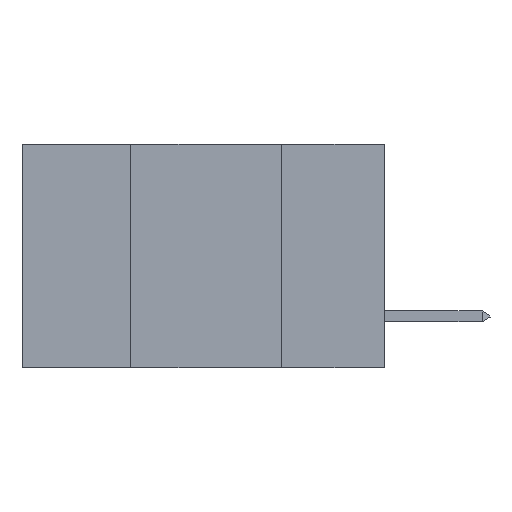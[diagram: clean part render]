
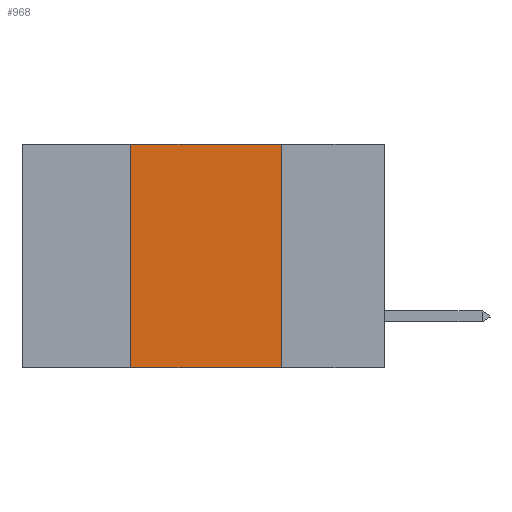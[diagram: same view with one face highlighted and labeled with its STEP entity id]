
A CAD part, left-side view. The second image highlights one B-rep face of the part: STEP entity #968.
In plain terms, the highlighted planar face has unit normal (-1, 0, 0).
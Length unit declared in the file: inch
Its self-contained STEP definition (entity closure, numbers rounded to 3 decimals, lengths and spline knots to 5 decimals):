
#968 = ADVANCED_FACE ( 'NONE', ( #14739 ), #27433, .F. ) ;
#1146 = EDGE_CURVE ( 'NONE', #17341, #30372, #25271, .T. ) ;
#1219 = CARTESIAN_POINT ( 'NONE',  ( 0., 0.42, -0.37 ) ) ;
#2249 = DIRECTION ( 'NONE',  ( 1., 0., 0. ) ) ;
#3747 = CARTESIAN_POINT ( 'NONE',  ( 0., 0.17, 0. ) ) ;
#4158 = DIRECTION ( 'NONE',  ( 0., -1., 0. ) ) ;
#4792 = DIRECTION ( 'NONE',  ( 0., 0., -1. ) ) ;
#5296 = LINE ( 'NONE', #9425, #22222 ) ;
#6341 = VERTEX_POINT ( 'NONE', #28883 ) ;
#7654 = ORIENTED_EDGE ( 'NONE', *, *, #20217, .T. ) ;
#8014 = CARTESIAN_POINT ( 'NONE',  ( 0., 0.42, 0. ) ) ;
#8727 = DIRECTION ( 'NONE',  ( 0., 0., 1. ) ) ;
#8892 = VECTOR ( 'NONE', #24467, 39.37008 ) ;
#9425 = CARTESIAN_POINT ( 'NONE',  ( 0., 0.6, -0.37 ) ) ;
#9540 = VERTEX_POINT ( 'NONE', #1219 ) ;
#10254 = CARTESIAN_POINT ( 'NONE',  ( 0., 0.6, 0. ) ) ;
#10966 = ORIENTED_EDGE ( 'NONE', *, *, #18745, .F. ) ;
#12131 = DIRECTION ( 'NONE',  ( 0., -1., 0. ) ) ;
#13094 = ORIENTED_EDGE ( 'NONE', *, *, #1146, .F. ) ;
#13785 = LINE ( 'NONE', #8014, #29041 ) ;
#14739 = FACE_OUTER_BOUND ( 'NONE', #22120, .T. ) ;
#14988 = LINE ( 'NONE', #26780, #16953 ) ;
#16953 = VECTOR ( 'NONE', #12131, 39.37008 ) ;
#17019 = CARTESIAN_POINT ( 'NONE',  ( 0., 0.17, -0.37 ) ) ;
#17341 = VERTEX_POINT ( 'NONE', #3747 ) ;
#18745 = EDGE_CURVE ( 'NONE', #6341, #17341, #14988, .T. ) ;
#19421 = AXIS2_PLACEMENT_3D ( 'NONE', #10254, #2249, #4792 ) ;
#19465 = EDGE_CURVE ( 'NONE', #9540, #6341, #13785, .T. ) ;
#20217 = EDGE_CURVE ( 'NONE', #9540, #30372, #5296, .T. ) ;
#22120 = EDGE_LOOP ( 'NONE', ( #13094, #10966, #24376, #7654 ) ) ;
#22222 = VECTOR ( 'NONE', #4158, 39.37008 ) ;
#24376 = ORIENTED_EDGE ( 'NONE', *, *, #19465, .F. ) ;
#24467 = DIRECTION ( 'NONE',  ( 0., 0., -1. ) ) ;
#25271 = LINE ( 'NONE', #26086, #8892 ) ;
#26086 = CARTESIAN_POINT ( 'NONE',  ( 0., 0.17, 0. ) ) ;
#26780 = CARTESIAN_POINT ( 'NONE',  ( 0., 0.6, 0. ) ) ;
#27433 = PLANE ( 'NONE',  #19421 ) ;
#28883 = CARTESIAN_POINT ( 'NONE',  ( 0., 0.42, 0. ) ) ;
#29041 = VECTOR ( 'NONE', #8727, 39.37008 ) ;
#30372 = VERTEX_POINT ( 'NONE', #17019 ) ;
